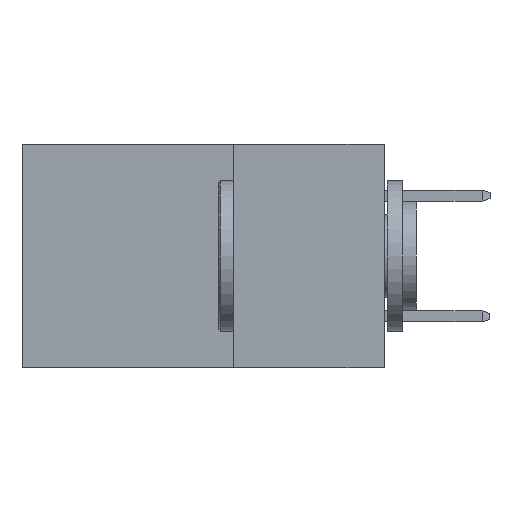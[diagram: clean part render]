
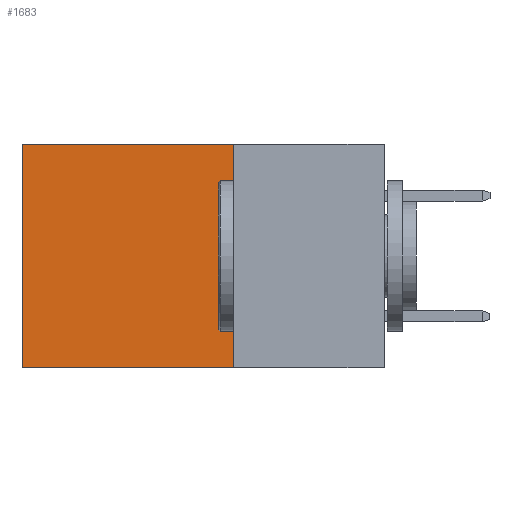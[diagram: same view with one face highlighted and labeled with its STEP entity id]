
A CAD part, left-side view. The second image highlights one B-rep face of the part: STEP entity #1683.
In plain terms, the highlighted planar face has unit normal (-1, 0, 0).
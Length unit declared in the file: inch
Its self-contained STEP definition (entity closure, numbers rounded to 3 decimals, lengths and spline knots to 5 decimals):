
#443 = VECTOR ( 'NONE', #4760, 39.37008 ) ;
#502 = ORIENTED_EDGE ( 'NONE', *, *, #8733, .T. ) ;
#511 = PLANE ( 'NONE',  #624 ) ;
#603 = FACE_OUTER_BOUND ( 'NONE', #13827, .T. ) ;
#624 = AXIS2_PLACEMENT_3D ( 'NONE', #2206, #9027, #1321 ) ;
#666 = LINE ( 'NONE', #14125, #12463 ) ;
#826 = ORIENTED_EDGE ( 'NONE', *, *, #14353, .T. ) ;
#1103 = VERTEX_POINT ( 'NONE', #18788 ) ;
#1321 = DIRECTION ( 'NONE',  ( 0., 0., -1. ) ) ;
#1683 = ADVANCED_FACE ( 'NONE', ( #603 ), #511, .F. ) ;
#2206 = CARTESIAN_POINT ( 'NONE',  ( 0.298, 0.25, 0. ) ) ;
#4087 = VERTEX_POINT ( 'NONE', #6663 ) ;
#4457 = CARTESIAN_POINT ( 'NONE',  ( 0.298, 0.6, -0.37 ) ) ;
#4760 = DIRECTION ( 'NONE',  ( 0., 0., -1. ) ) ;
#5022 = CARTESIAN_POINT ( 'NONE',  ( 0.298, 0.6, 0. ) ) ;
#5488 = VERTEX_POINT ( 'NONE', #4457 ) ;
#6329 = VERTEX_POINT ( 'NONE', #19267 ) ;
#6663 = CARTESIAN_POINT ( 'NONE',  ( 0.298, 0.6, 0. ) ) ;
#8025 = DIRECTION ( 'NONE',  ( 0., 0., -1. ) ) ;
#8252 = EDGE_CURVE ( 'NONE', #6329, #5488, #666, .T. ) ;
#8733 = EDGE_CURVE ( 'NONE', #4087, #5488, #17128, .T. ) ;
#9027 = DIRECTION ( 'NONE',  ( 1., 0., 0. ) ) ;
#10932 = ORIENTED_EDGE ( 'NONE', *, *, #14898, .F. ) ;
#12463 = VECTOR ( 'NONE', #13942, 39.37008 ) ;
#13004 = CARTESIAN_POINT ( 'NONE',  ( 0.298, 0.25, 0. ) ) ;
#13383 = VECTOR ( 'NONE', #8025, 39.37008 ) ;
#13827 = EDGE_LOOP ( 'NONE', ( #502, #15604, #10932, #826 ) ) ;
#13942 = DIRECTION ( 'NONE',  ( 0., 1., 0. ) ) ;
#14125 = CARTESIAN_POINT ( 'NONE',  ( 0.298, 0.25, -0.37 ) ) ;
#14353 = EDGE_CURVE ( 'NONE', #1103, #4087, #15306, .T. ) ;
#14500 = DIRECTION ( 'NONE',  ( 0., 1., 0. ) ) ;
#14898 = EDGE_CURVE ( 'NONE', #1103, #6329, #17812, .T. ) ;
#15306 = LINE ( 'NONE', #13004, #19266 ) ;
#15604 = ORIENTED_EDGE ( 'NONE', *, *, #8252, .F. ) ;
#17128 = LINE ( 'NONE', #5022, #443 ) ;
#17812 = LINE ( 'NONE', #18577, #13383 ) ;
#18577 = CARTESIAN_POINT ( 'NONE',  ( 0.298, 0.25, 0. ) ) ;
#18788 = CARTESIAN_POINT ( 'NONE',  ( 0.298, 0.25, 0. ) ) ;
#19266 = VECTOR ( 'NONE', #14500, 39.37008 ) ;
#19267 = CARTESIAN_POINT ( 'NONE',  ( 0.298, 0.25, -0.37 ) ) ;
